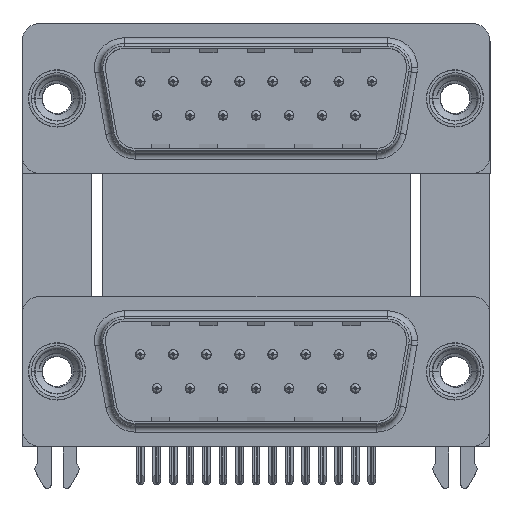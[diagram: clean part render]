
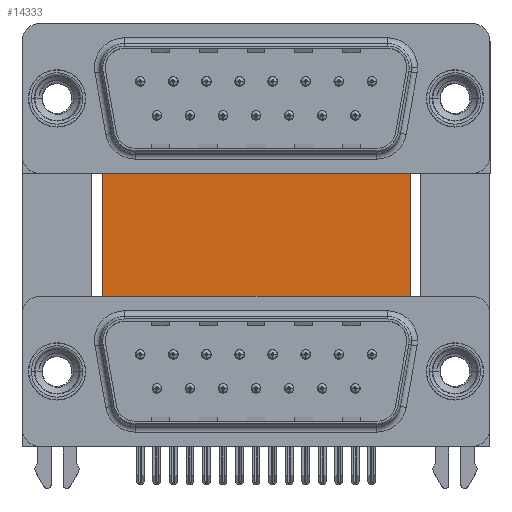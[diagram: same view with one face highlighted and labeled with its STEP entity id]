
A CAD part, top view. The second image highlights one B-rep face of the part: STEP entity #14333.
In plain terms, the highlighted planar face has unit normal (0, 0, 1).
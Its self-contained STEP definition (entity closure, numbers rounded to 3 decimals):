
#1005 = DIRECTION ( 'NONE',  ( -1., 0., 0. ) ) ;
#2846 = AXIS2_PLACEMENT_3D ( 'NONE', #8765, #32183, #1005 ) ;
#3284 = CARTESIAN_POINT ( 'NONE',  ( 3.79, -3.735, -12. ) ) ;
#3889 = FACE_OUTER_BOUND ( 'NONE', #29180, .T. ) ;
#4387 = VERTEX_POINT ( 'NONE', #15122 ) ;
#6333 = EDGE_CURVE ( 'NONE', #30384, #17166, #10620, .T. ) ;
#8765 = CARTESIAN_POINT ( 'NONE',  ( 3.79, 16.585, -12. ) ) ;
#10620 = LINE ( 'NONE', #11309, #15072 ) ;
#11309 = CARTESIAN_POINT ( 'NONE',  ( 3.79, -3.735, -12. ) ) ;
#11429 = DIRECTION ( 'NONE',  ( 0., -1., 0. ) ) ;
#11639 = DIRECTION ( 'NONE',  ( 1., 0., 0. ) ) ;
#12245 = LINE ( 'NONE', #22760, #27764 ) ;
#13044 = ORIENTED_EDGE ( 'NONE', *, *, #25296, .F. ) ;
#13427 = CARTESIAN_POINT ( 'NONE',  ( 29.58, 16.585, -12. ) ) ;
#13514 = EDGE_CURVE ( 'NONE', #4387, #30384, #32944, .T. ) ;
#14333 = ADVANCED_FACE ( 'NONE', ( #3889 ), #31503, .F. ) ;
#15072 = VECTOR ( 'NONE', #11639, 1000. ) ;
#15122 = CARTESIAN_POINT ( 'NONE',  ( 3.79, 16.585, -12. ) ) ;
#15407 = ORIENTED_EDGE ( 'NONE', *, *, #13514, .T. ) ;
#15850 = LINE ( 'NONE', #13427, #32133 ) ;
#17160 = ORIENTED_EDGE ( 'NONE', *, *, #21081, .F. ) ;
#17166 = VERTEX_POINT ( 'NONE', #30929 ) ;
#20177 = DIRECTION ( 'NONE',  ( 1., 0., 0. ) ) ;
#21081 = EDGE_CURVE ( 'NONE', #22978, #17166, #15850, .T. ) ;
#22760 = CARTESIAN_POINT ( 'NONE',  ( 3.79, 16.585, -12. ) ) ;
#22978 = VERTEX_POINT ( 'NONE', #26478 ) ;
#24301 = VECTOR ( 'NONE', #11429, 1000. ) ;
#24878 = CARTESIAN_POINT ( 'NONE',  ( 3.79, 16.585, -12. ) ) ;
#25296 = EDGE_CURVE ( 'NONE', #4387, #22978, #12245, .T. ) ;
#26478 = CARTESIAN_POINT ( 'NONE',  ( 29.58, 16.585, -12. ) ) ;
#27764 = VECTOR ( 'NONE', #20177, 1000. ) ;
#29180 = EDGE_LOOP ( 'NONE', ( #32469, #17160, #13044, #15407 ) ) ;
#30384 = VERTEX_POINT ( 'NONE', #3284 ) ;
#30929 = CARTESIAN_POINT ( 'NONE',  ( 29.58, -3.735, -12. ) ) ;
#31503 = PLANE ( 'NONE',  #2846 ) ;
#31665 = DIRECTION ( 'NONE',  ( 0., -1., 0. ) ) ;
#32133 = VECTOR ( 'NONE', #31665, 1000. ) ;
#32183 = DIRECTION ( 'NONE',  ( 0., 0., -1. ) ) ;
#32469 = ORIENTED_EDGE ( 'NONE', *, *, #6333, .T. ) ;
#32944 = LINE ( 'NONE', #24878, #24301 ) ;
